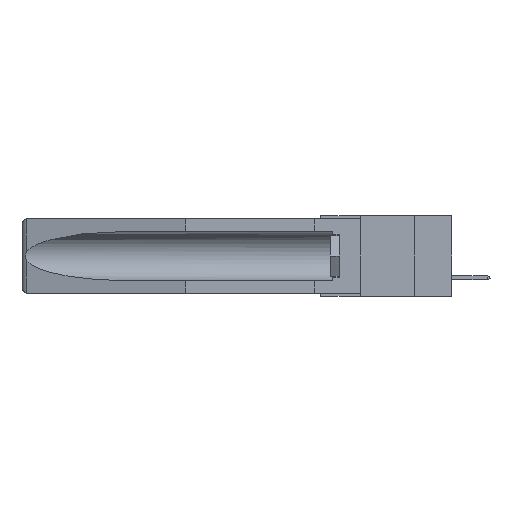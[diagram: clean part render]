
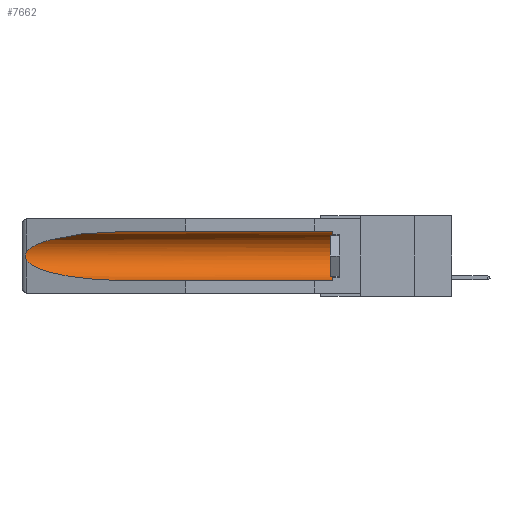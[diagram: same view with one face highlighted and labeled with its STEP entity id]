
A CAD part, left-side view. The second image highlights one B-rep face of the part: STEP entity #7662.
In plain terms, the highlighted cylindrical face has radius 2.857 mm (diameter 5.715 mm), a partial arc.
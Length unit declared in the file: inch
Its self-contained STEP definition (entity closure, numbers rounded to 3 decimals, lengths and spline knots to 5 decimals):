
#283 = EDGE_CURVE ( 'NONE', #12010, #21186, #20005, .T. ) ;
#1315 = ORIENTED_EDGE ( 'NONE', *, *, #283, .T. ) ;
#2852 = CARTESIAN_POINT ( 'NONE',  ( 0.26537, 1.52718, -0.19328 ) ) ;
#2993 = CARTESIAN_POINT ( 'NONE',  ( 0.155, 0.126, -0.1715 ) ) ;
#3292 = ORIENTED_EDGE ( 'NONE', *, *, #18862, .T. ) ;
#3324 =( BOUNDED_CURVE ( )  B_SPLINE_CURVE ( 3, ( #22776, #7207, #19214, #5400 ),
 .UNSPECIFIED., .F., .F. ) 
 B_SPLINE_CURVE_WITH_KNOTS ( ( 4, 4 ),
 ( 0.1948, 1.5708 ),
 .UNSPECIFIED. ) 
 CURVE ( )  GEOMETRIC_REPRESENTATION_ITEM ( )  RATIONAL_B_SPLINE_CURVE ( ( 1., 0.848, 0.848, 1. ) ) 
 REPRESENTATION_ITEM ( '' )  );
#3531 = EDGE_CURVE ( 'NONE', #21186, #19481, #11565, .T. ) ;
#4540 = CARTESIAN_POINT ( 'NONE',  ( 0.2675, 1.53308, -0.17534 ) ) ;
#4991 = CARTESIAN_POINT ( 'NONE',  ( 0.155, 1.07973, -0.059 ) ) ;
#5400 = CARTESIAN_POINT ( 'NONE',  ( 0.155, 1.07973, -0.284 ) ) ;
#5521 = DIRECTION ( 'NONE',  ( 0., 1., 0. ) ) ;
#6168 = CARTESIAN_POINT ( 'NONE',  ( 0.2675, 1.53308, -0.16763 ) ) ;
#6877 = EDGE_CURVE ( 'NONE', #19706, #12010, #15433, .T. ) ;
#7207 = CARTESIAN_POINT ( 'NONE',  ( 0.25451, 1.48313, -0.24835 ) ) ;
#7662 = ADVANCED_FACE ( 'NONE', ( #21148 ), #14017, .F. ) ;
#7680 = CARTESIAN_POINT ( 'NONE',  ( 0.26537, 1.52718, -0.14972 ) ) ;
#7759 = ORIENTED_EDGE ( 'NONE', *, *, #6877, .T. ) ;
#7859 = CIRCLE ( 'NONE', #13469, 0.1125 ) ;
#8116 = CARTESIAN_POINT ( 'NONE',  ( 0.155, 1.07973, -0.284 ) ) ;
#8125 = CARTESIAN_POINT ( 'NONE',  ( 0.2673, 1.5327, -0.16383 ) ) ;
#8211 = CARTESIAN_POINT ( 'NONE',  ( 0.2673, 1.53269, -0.17917 ) ) ;
#8689 = LINE ( 'NONE', #21259, #14756 ) ;
#9830 = CARTESIAN_POINT ( 'NONE',  ( 0.155, 0.126, -0.059 ) ) ;
#9900 = DIRECTION ( 'NONE',  ( 0., 0., 1. ) ) ;
#10042 = VERTEX_POINT ( 'NONE', #19253 ) ;
#10284 = CARTESIAN_POINT ( 'NONE',  ( 0.25451, 1.48313, -0.09465 ) ) ;
#11023 = VECTOR ( 'NONE', #11091, 39.37008 ) ;
#11074 = EDGE_CURVE ( 'NONE', #10042, #17351, #8689, .T. ) ;
#11091 = DIRECTION ( 'NONE',  ( 0., 1., 0. ) ) ;
#11565 = B_SPLINE_CURVE_WITH_KNOTS ( 'NONE', 3,
 ( #7680, #13097, #15293, #8125, #6168, #4540, #8211, #13550, #16891, #2852 ),
 .UNSPECIFIED., .F., .F.,
 ( 4, 2, 2, 2, 4 ),
 ( 0., 0.00029, 0.00058, 0.00087, 0.00117 ),
 .UNSPECIFIED. ) ;
#12010 = VERTEX_POINT ( 'NONE', #17766 ) ;
#13097 = CARTESIAN_POINT ( 'NONE',  ( 0.26597, 1.52961, -0.15275 ) ) ;
#13469 = AXIS2_PLACEMENT_3D ( 'NONE', #2993, #14852, #9900 ) ;
#13550 = CARTESIAN_POINT ( 'NONE',  ( 0.26655, 1.53094, -0.18657 ) ) ;
#13664 = EDGE_CURVE ( 'NONE', #19481, #17351, #3324, .T. ) ;
#13669 = EDGE_LOOP ( 'NONE', ( #1315, #19606, #21125, #16371, #3292, #7759 ) ) ;
#13910 = CARTESIAN_POINT ( 'NONE',  ( 0.21114, 1.30732, -0.059 ) ) ;
#14017 = CYLINDRICAL_SURFACE ( 'NONE', #21540, 0.1125 ) ;
#14479 = CARTESIAN_POINT ( 'NONE',  ( 0.155, -0.30754, -0.1715 ) ) ;
#14639 = CARTESIAN_POINT ( 'NONE',  ( 0.155, -0.30754, -0.059 ) ) ;
#14756 = VECTOR ( 'NONE', #5521, 39.37008 ) ;
#14852 = DIRECTION ( 'NONE',  ( 0., -1., 0. ) ) ;
#15293 = CARTESIAN_POINT ( 'NONE',  ( 0.26654, 1.53092, -0.15636 ) ) ;
#15433 = LINE ( 'NONE', #14639, #11023 ) ;
#15667 = CARTESIAN_POINT ( 'NONE',  ( 0.26537, 1.52718, -0.14972 ) ) ;
#16151 = CARTESIAN_POINT ( 'NONE',  ( 0.26537, 1.52718, -0.14972 ) ) ;
#16371 = ORIENTED_EDGE ( 'NONE', *, *, #11074, .F. ) ;
#16582 = CARTESIAN_POINT ( 'NONE',  ( 0.26537, 1.52718, -0.19328 ) ) ;
#16891 = CARTESIAN_POINT ( 'NONE',  ( 0.26597, 1.5296, -0.19026 ) ) ;
#17351 = VERTEX_POINT ( 'NONE', #8116 ) ;
#17766 = CARTESIAN_POINT ( 'NONE',  ( 0.155, 1.07973, -0.059 ) ) ;
#18862 = EDGE_CURVE ( 'NONE', #10042, #19706, #7859, .T. ) ;
#19214 = CARTESIAN_POINT ( 'NONE',  ( 0.21114, 1.30732, -0.284 ) ) ;
#19253 = CARTESIAN_POINT ( 'NONE',  ( 0.155, 0.126, -0.284 ) ) ;
#19471 = DIRECTION ( 'NONE',  ( 0., 1., 0. ) ) ;
#19481 = VERTEX_POINT ( 'NONE', #16582 ) ;
#19547 = DIRECTION ( 'NONE',  ( 0., 0., 1. ) ) ;
#19606 = ORIENTED_EDGE ( 'NONE', *, *, #3531, .T. ) ;
#19706 = VERTEX_POINT ( 'NONE', #9830 ) ;
#20005 =( BOUNDED_CURVE ( )  B_SPLINE_CURVE ( 3, ( #4991, #13910, #10284, #15667 ),
 .UNSPECIFIED., .F., .F. ) 
 B_SPLINE_CURVE_WITH_KNOTS ( ( 4, 4 ),
 ( 4.71239, 6.08839 ),
 .UNSPECIFIED. ) 
 CURVE ( )  GEOMETRIC_REPRESENTATION_ITEM ( )  RATIONAL_B_SPLINE_CURVE ( ( 1., 0.848, 0.848, 1. ) ) 
 REPRESENTATION_ITEM ( '' )  );
#21125 = ORIENTED_EDGE ( 'NONE', *, *, #13664, .T. ) ;
#21148 = FACE_OUTER_BOUND ( 'NONE', #13669, .T. ) ;
#21186 = VERTEX_POINT ( 'NONE', #16151 ) ;
#21259 = CARTESIAN_POINT ( 'NONE',  ( 0.155, -0.30754, -0.284 ) ) ;
#21540 = AXIS2_PLACEMENT_3D ( 'NONE', #14479, #19471, #19547 ) ;
#22776 = CARTESIAN_POINT ( 'NONE',  ( 0.26537, 1.52718, -0.19328 ) ) ;
